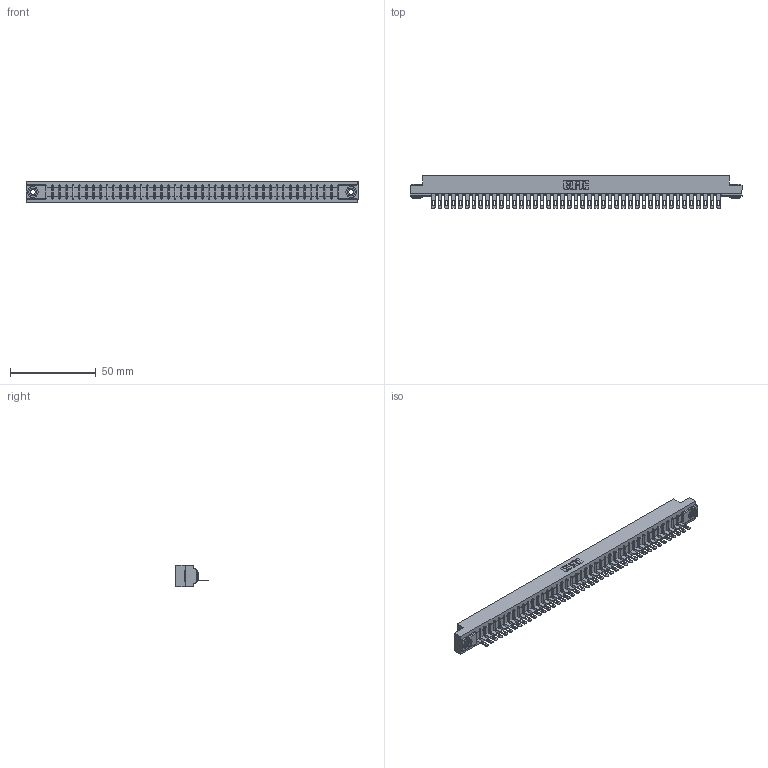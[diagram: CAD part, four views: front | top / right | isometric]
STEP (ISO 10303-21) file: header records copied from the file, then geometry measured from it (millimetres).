
FILE_DESCRIPTION (( 'STEP AP203' ), '1' );
FILE_NAME ('357-043-505-103.STEP', '2019-09-14T16:30:51', ( '' ), ( '' ), 'SwSTEP 2.0', 'SolidWorks 2016', '' );
FILE_SCHEMA (( 'CONFIG_CONTROL_DESIGN' ));
Length unit declared in the file: inch
Products named in the file (4): 345-250-002_345-250-002-102; 357-043-505-103; 307 Part_.156 Dia Mounting Holes; 307-290-001_505
Assembly tree (46 placements, depth 2):
  357-043-505-103
    307 Part_.156 Dia Mounting Holes
    307-290-001_505  x43
    345-250-002_345-250-002-102  x2
Bounding box: 193.4 x 19.18 x 12.7 mm (x, y, z)
Volume: 20142.2 mm3; surface area: 21958 mm2
Topology: 46 solids, 46 shells, 2622 faces, 7401 edges, 4754 vertices
Faces by surface type: plane 1642, cylinder 884, sphere 88, cone 8
Entity records: 37779 total; most frequent: CARTESIAN_POINT 6341, ORIENTED_EDGE 6318, DIRECTION 6183, EDGE_CURVE 3159, VECTOR 2415, LINE 2415, VERTEX_POINT 2042, AXIS2_PLACEMENT_3D 1884
